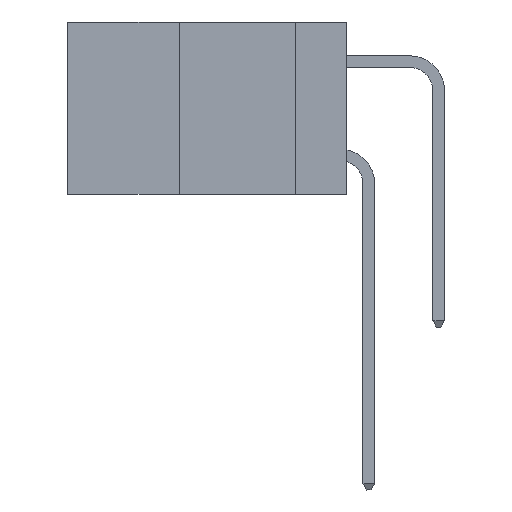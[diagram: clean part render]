
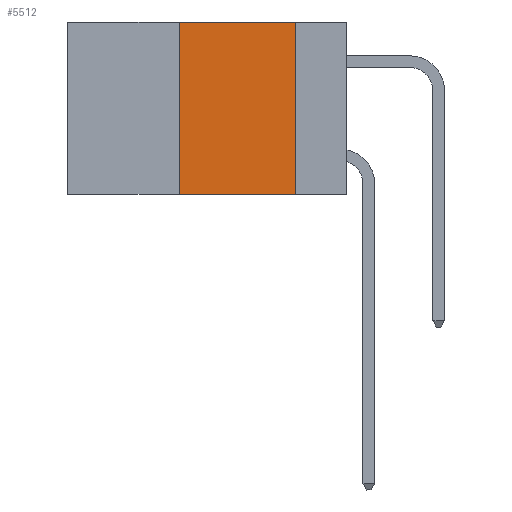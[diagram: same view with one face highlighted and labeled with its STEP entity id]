
A CAD part, left-side view. The second image highlights one B-rep face of the part: STEP entity #5512.
In plain terms, the highlighted planar face has unit normal (-1, 0, 0).
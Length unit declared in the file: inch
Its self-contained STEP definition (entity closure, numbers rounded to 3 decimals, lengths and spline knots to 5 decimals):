
#688 = DIRECTION ( 'NONE',  ( 0., 0., 1. ) ) ;
#790 = VECTOR ( 'NONE', #4061, 39.37008 ) ;
#805 = DIRECTION ( 'NONE',  ( 1., 0., 0. ) ) ;
#1325 = LINE ( 'NONE', #6527, #790 ) ;
#1537 = EDGE_CURVE ( 'NONE', #8670, #7702, #8087, .T. ) ;
#1655 = AXIS2_PLACEMENT_3D ( 'NONE', #5768, #805, #3398 ) ;
#1864 = VERTEX_POINT ( 'NONE', #10356 ) ;
#1999 = CARTESIAN_POINT ( 'NONE',  ( 0., 0.11, 0. ) ) ;
#2179 = CARTESIAN_POINT ( 'NONE',  ( 0., 0.36, 0. ) ) ;
#2430 = VECTOR ( 'NONE', #688, 39.37008 ) ;
#2936 = VECTOR ( 'NONE', #7122, 39.37008 ) ;
#3398 = DIRECTION ( 'NONE',  ( 0., 0., -1. ) ) ;
#3554 = EDGE_CURVE ( 'NONE', #1864, #8670, #1325, .T. ) ;
#3996 = ORIENTED_EDGE ( 'NONE', *, *, #3554, .F. ) ;
#4061 = DIRECTION ( 'NONE',  ( 0., -1., 0. ) ) ;
#4902 = DIRECTION ( 'NONE',  ( 0., 0., -1. ) ) ;
#4905 = FACE_OUTER_BOUND ( 'NONE', #8943, .T. ) ;
#4934 = CARTESIAN_POINT ( 'NONE',  ( 0., 0.11, 0. ) ) ;
#5263 = VECTOR ( 'NONE', #4902, 39.37008 ) ;
#5512 = ADVANCED_FACE ( 'NONE', ( #4905 ), #7384, .F. ) ;
#5530 = LINE ( 'NONE', #7190, #2936 ) ;
#5662 = EDGE_CURVE ( 'NONE', #7552, #1864, #7479, .T. ) ;
#5768 = CARTESIAN_POINT ( 'NONE',  ( 0., 0.6, 0. ) ) ;
#6527 = CARTESIAN_POINT ( 'NONE',  ( 0., 0.6, 0. ) ) ;
#7122 = DIRECTION ( 'NONE',  ( 0., -1., 0. ) ) ;
#7190 = CARTESIAN_POINT ( 'NONE',  ( 0., 0.6, -0.37 ) ) ;
#7384 = PLANE ( 'NONE',  #1655 ) ;
#7479 = LINE ( 'NONE', #2179, #2430 ) ;
#7552 = VERTEX_POINT ( 'NONE', #8446 ) ;
#7702 = VERTEX_POINT ( 'NONE', #9658 ) ;
#8087 = LINE ( 'NONE', #4934, #5263 ) ;
#8446 = CARTESIAN_POINT ( 'NONE',  ( 0., 0.36, -0.37 ) ) ;
#8670 = VERTEX_POINT ( 'NONE', #1999 ) ;
#8943 = EDGE_LOOP ( 'NONE', ( #10314, #3996, #9124, #9269 ) ) ;
#9007 = EDGE_CURVE ( 'NONE', #7552, #7702, #5530, .T. ) ;
#9124 = ORIENTED_EDGE ( 'NONE', *, *, #5662, .F. ) ;
#9269 = ORIENTED_EDGE ( 'NONE', *, *, #9007, .T. ) ;
#9658 = CARTESIAN_POINT ( 'NONE',  ( 0., 0.11, -0.37 ) ) ;
#10314 = ORIENTED_EDGE ( 'NONE', *, *, #1537, .F. ) ;
#10356 = CARTESIAN_POINT ( 'NONE',  ( 0., 0.36, 0. ) ) ;
